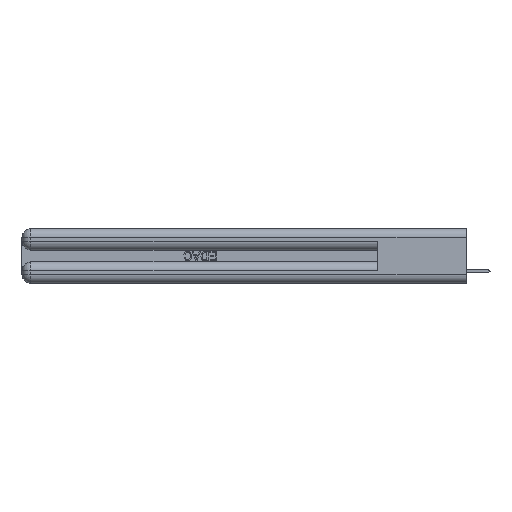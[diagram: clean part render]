
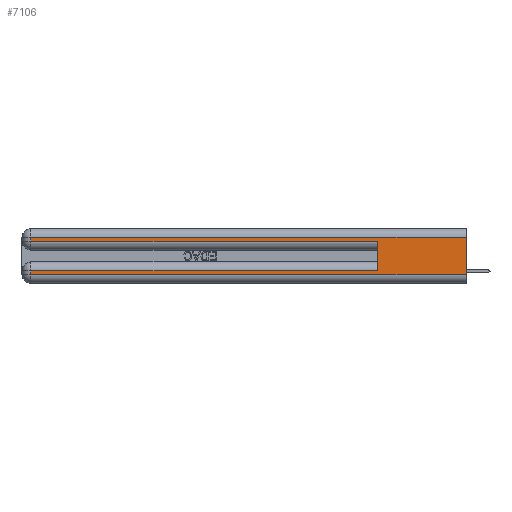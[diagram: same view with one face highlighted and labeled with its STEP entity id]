
A CAD part, left-side view. The second image highlights one B-rep face of the part: STEP entity #7106.
In plain terms, the highlighted planar face has unit normal (-1, 0, 0).
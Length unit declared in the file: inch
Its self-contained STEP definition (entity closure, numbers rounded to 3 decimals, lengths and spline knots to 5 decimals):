
#54 = ORIENTED_EDGE ( 'NONE', *, *, #18544, .T. ) ;
#446 = VECTOR ( 'NONE', #49316, 39.37008 ) ;
#1458 = LINE ( 'NONE', #40599, #48168 ) ;
#3848 = ORIENTED_EDGE ( 'NONE', *, *, #12060, .T. ) ;
#5123 = LINE ( 'NONE', #34270, #46508 ) ;
#5128 = VECTOR ( 'NONE', #10055, 39.37008 ) ;
#5737 = LINE ( 'NONE', #9991, #48564 ) ;
#6005 = CARTESIAN_POINT ( 'NONE',  ( 0., 2.94, 0.37 ) ) ;
#7106 = ADVANCED_FACE ( 'NONE', ( #45022 ), #26905, .F. ) ;
#7763 = EDGE_CURVE ( 'NONE', #18660, #31242, #1458, .T. ) ;
#8203 = CARTESIAN_POINT ( 'NONE',  ( 0., 2.94, 0.085 ) ) ;
#8618 = VERTEX_POINT ( 'NONE', #35997 ) ;
#9991 = CARTESIAN_POINT ( 'NONE',  ( 0., 0., 0.285 ) ) ;
#10055 = DIRECTION ( 'NONE',  ( 0., 0., -1. ) ) ;
#10189 = ORIENTED_EDGE ( 'NONE', *, *, #44826, .F. ) ;
#12060 = EDGE_CURVE ( 'NONE', #41707, #42218, #26890, .T. ) ;
#12249 = VERTEX_POINT ( 'NONE', #34969 ) ;
#13625 = DIRECTION ( 'NONE',  ( 0., -1., 0. ) ) ;
#13740 = VERTEX_POINT ( 'NONE', #14220 ) ;
#14220 = CARTESIAN_POINT ( 'NONE',  ( 0., 0.6, 0.285 ) ) ;
#15071 = CARTESIAN_POINT ( 'NONE',  ( 0., 0., 0.31 ) ) ;
#15077 = DIRECTION ( 'NONE',  ( 0., 0., -1. ) ) ;
#15172 = DIRECTION ( 'NONE',  ( 0., 1., 0. ) ) ;
#16223 = ORIENTED_EDGE ( 'NONE', *, *, #16425, .T. ) ;
#16425 = EDGE_CURVE ( 'NONE', #49945, #41707, #29887, .T. ) ;
#18544 = EDGE_CURVE ( 'NONE', #31242, #12249, #5123, .T. ) ;
#18581 = CARTESIAN_POINT ( 'NONE',  ( 0., 0.6, 0.145 ) ) ;
#18660 = VERTEX_POINT ( 'NONE', #15071 ) ;
#18995 = VECTOR ( 'NONE', #15172, 39.37008 ) ;
#19269 = CARTESIAN_POINT ( 'NONE',  ( 0., 2.94, 0.06 ) ) ;
#23349 = DIRECTION ( 'NONE',  ( 1., 0., 0. ) ) ;
#24008 = ORIENTED_EDGE ( 'NONE', *, *, #36831, .T. ) ;
#26890 = LINE ( 'NONE', #6005, #47634 ) ;
#26905 = PLANE ( 'NONE',  #47176 ) ;
#28663 = VECTOR ( 'NONE', #35197, 39.37008 ) ;
#29887 = LINE ( 'NONE', #52004, #18995 ) ;
#31188 = LINE ( 'NONE', #18581, #28663 ) ;
#31242 = VERTEX_POINT ( 'NONE', #39466 ) ;
#33585 = DIRECTION ( 'NONE',  ( 0., 0., -1. ) ) ;
#34270 = CARTESIAN_POINT ( 'NONE',  ( 0., 2.94, 0.37 ) ) ;
#34915 = DIRECTION ( 'NONE',  ( 0., 0., -1. ) ) ;
#34969 = CARTESIAN_POINT ( 'NONE',  ( 0., 2.94, 0.285 ) ) ;
#35197 = DIRECTION ( 'NONE',  ( 0., 0., 1. ) ) ;
#35997 = CARTESIAN_POINT ( 'NONE',  ( 0., 0., 0.06 ) ) ;
#36831 = EDGE_CURVE ( 'NONE', #42218, #8618, #49096, .T. ) ;
#37355 = ORIENTED_EDGE ( 'NONE', *, *, #40823, .F. ) ;
#38406 = CARTESIAN_POINT ( 'NONE',  ( 0., 0.6, 0.085 ) ) ;
#39120 = CARTESIAN_POINT ( 'NONE',  ( 0., 0., 0.37 ) ) ;
#39466 = CARTESIAN_POINT ( 'NONE',  ( 0., 2.94, 0.31 ) ) ;
#40599 = CARTESIAN_POINT ( 'NONE',  ( 0., 0., 0.31 ) ) ;
#40823 = EDGE_CURVE ( 'NONE', #18660, #8618, #42033, .T. ) ;
#40975 = CARTESIAN_POINT ( 'NONE',  ( 0., 0., 0.06 ) ) ;
#41151 = ORIENTED_EDGE ( 'NONE', *, *, #7763, .T. ) ;
#41223 = EDGE_CURVE ( 'NONE', #12249, #13740, #5737, .T. ) ;
#41707 = VERTEX_POINT ( 'NONE', #8203 ) ;
#42033 = LINE ( 'NONE', #39120, #5128 ) ;
#42218 = VERTEX_POINT ( 'NONE', #19269 ) ;
#43422 = EDGE_LOOP ( 'NONE', ( #37355, #41151, #54, #45465, #10189, #16223, #3848, #24008 ) ) ;
#44826 = EDGE_CURVE ( 'NONE', #49945, #13740, #31188, .T. ) ;
#45022 = FACE_OUTER_BOUND ( 'NONE', #43422, .T. ) ;
#45465 = ORIENTED_EDGE ( 'NONE', *, *, #41223, .T. ) ;
#46508 = VECTOR ( 'NONE', #33585, 39.37008 ) ;
#47176 = AXIS2_PLACEMENT_3D ( 'NONE', #47949, #23349, #15077 ) ;
#47634 = VECTOR ( 'NONE', #34915, 39.37008 ) ;
#47949 = CARTESIAN_POINT ( 'NONE',  ( 0., 0., 0.37 ) ) ;
#48168 = VECTOR ( 'NONE', #53088, 39.37008 ) ;
#48564 = VECTOR ( 'NONE', #13625, 39.37008 ) ;
#49096 = LINE ( 'NONE', #40975, #446 ) ;
#49316 = DIRECTION ( 'NONE',  ( 0., -1., 0. ) ) ;
#49945 = VERTEX_POINT ( 'NONE', #38406 ) ;
#52004 = CARTESIAN_POINT ( 'NONE',  ( 0., 0., 0.085 ) ) ;
#53088 = DIRECTION ( 'NONE',  ( 0., 1., 0. ) ) ;
